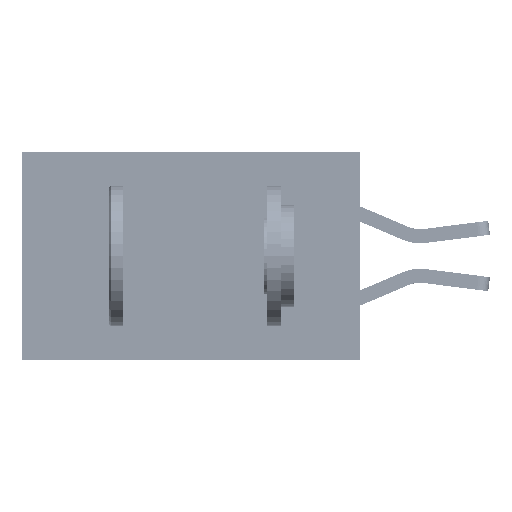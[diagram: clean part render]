
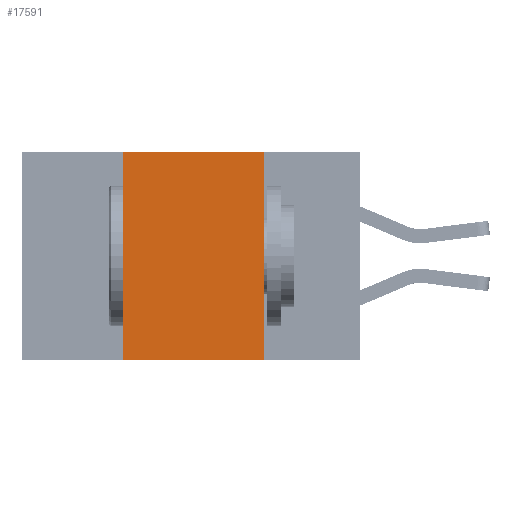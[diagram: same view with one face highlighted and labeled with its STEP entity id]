
A CAD part, left-side view. The second image highlights one B-rep face of the part: STEP entity #17591.
In plain terms, the highlighted planar face has unit normal (-1, 0, 0).
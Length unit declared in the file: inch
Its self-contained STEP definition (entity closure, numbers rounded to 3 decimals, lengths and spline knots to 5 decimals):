
#331 = CARTESIAN_POINT ( 'NONE',  ( 0., 0.6, 0. ) ) ;
#1491 = LINE ( 'NONE', #12115, #28930 ) ;
#2181 = VERTEX_POINT ( 'NONE', #3581 ) ;
#2461 = LINE ( 'NONE', #22792, #29511 ) ;
#2740 = VECTOR ( 'NONE', #38475, 39.37008 ) ;
#3581 = CARTESIAN_POINT ( 'NONE',  ( 0., 0.42, 0. ) ) ;
#5856 = FACE_OUTER_BOUND ( 'NONE', #11971, .T. ) ;
#7973 = LINE ( 'NONE', #331, #12464 ) ;
#9376 = ORIENTED_EDGE ( 'NONE', *, *, #26769, .T. ) ;
#11971 = EDGE_LOOP ( 'NONE', ( #15243, #24619, #39765, #9376 ) ) ;
#12115 = CARTESIAN_POINT ( 'NONE',  ( 0., 0.42, 0. ) ) ;
#12464 = VECTOR ( 'NONE', #22303, 39.37008 ) ;
#12790 = CARTESIAN_POINT ( 'NONE',  ( 0., 0.17, -0.37 ) ) ;
#13550 = DIRECTION ( 'NONE',  ( 1., 0., 0. ) ) ;
#14164 = EDGE_CURVE ( 'NONE', #30631, #35398, #40063, .T. ) ;
#15243 = ORIENTED_EDGE ( 'NONE', *, *, #14164, .F. ) ;
#17591 = ADVANCED_FACE ( 'NONE', ( #5856 ), #32525, .F. ) ;
#20862 = VERTEX_POINT ( 'NONE', #35717 ) ;
#22303 = DIRECTION ( 'NONE',  ( 0., -1., 0. ) ) ;
#22792 = CARTESIAN_POINT ( 'NONE',  ( 0., 0.6, -0.37 ) ) ;
#24619 = ORIENTED_EDGE ( 'NONE', *, *, #34546, .F. ) ;
#26769 = EDGE_CURVE ( 'NONE', #20862, #35398, #2461, .T. ) ;
#26949 = DIRECTION ( 'NONE',  ( 0., -1., 0. ) ) ;
#27161 = EDGE_CURVE ( 'NONE', #20862, #2181, #1491, .T. ) ;
#28930 = VECTOR ( 'NONE', #30667, 39.37008 ) ;
#29063 = CARTESIAN_POINT ( 'NONE',  ( 0., 0.6, 0. ) ) ;
#29511 = VECTOR ( 'NONE', #26949, 39.37008 ) ;
#29531 = CARTESIAN_POINT ( 'NONE',  ( 0., 0.17, 0. ) ) ;
#30631 = VERTEX_POINT ( 'NONE', #29531 ) ;
#30642 = CARTESIAN_POINT ( 'NONE',  ( 0., 0.17, 0. ) ) ;
#30667 = DIRECTION ( 'NONE',  ( 0., 0., 1. ) ) ;
#31969 = DIRECTION ( 'NONE',  ( 0., 0., -1. ) ) ;
#32525 = PLANE ( 'NONE',  #39771 ) ;
#34546 = EDGE_CURVE ( 'NONE', #2181, #30631, #7973, .T. ) ;
#35398 = VERTEX_POINT ( 'NONE', #12790 ) ;
#35717 = CARTESIAN_POINT ( 'NONE',  ( 0., 0.42, -0.37 ) ) ;
#38475 = DIRECTION ( 'NONE',  ( 0., 0., -1. ) ) ;
#39765 = ORIENTED_EDGE ( 'NONE', *, *, #27161, .F. ) ;
#39771 = AXIS2_PLACEMENT_3D ( 'NONE', #29063, #13550, #31969 ) ;
#40063 = LINE ( 'NONE', #30642, #2740 ) ;
